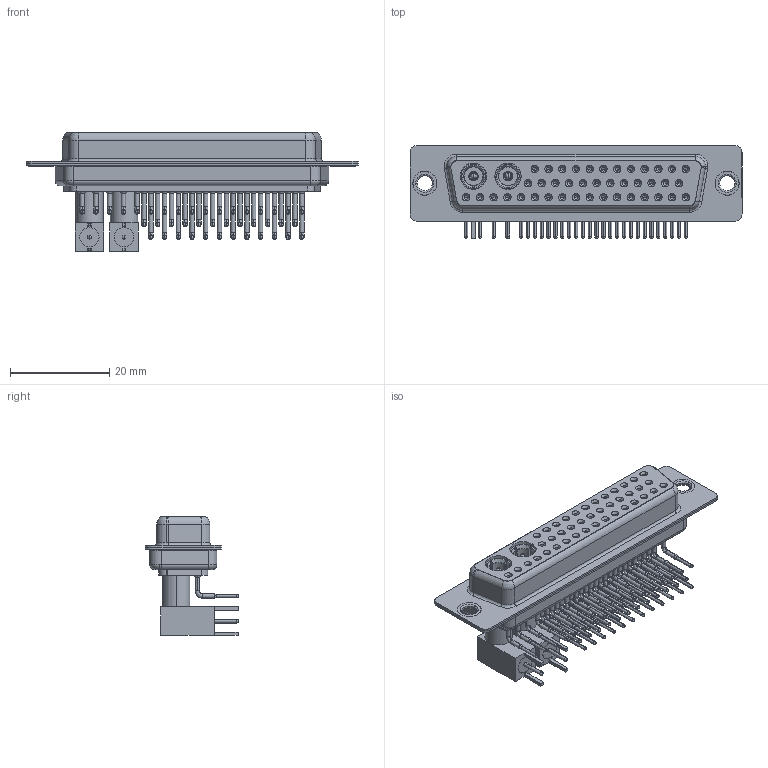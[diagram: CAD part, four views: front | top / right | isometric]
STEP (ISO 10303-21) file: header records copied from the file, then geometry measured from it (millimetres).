
FILE_DESCRIPTION (( 'STEP AP203' ), '1' );
FILE_NAME ('630-43W2240-7T1.STEP', '2022-06-09T19:07:29', ( '' ), ( '' ), 'SwSTEP 2.0', 'SolidWorks 2020', '' );
FILE_SCHEMA (( 'CONFIG_CONTROL_DESIGN' ));
Length unit declared in the file: millimetre
Products named in the file (16): 630Combo Housing_43W2; Locking Collar; Insulator RA Pin; 630Combo Thru Hole Rivet; Co-Ax Plug_RA 50; 630Combo Shell Rear_50 Contacts; 630-43W2240-7T1; 630Combo Shell Front_50 Contacts; RA Back Shell_50; Insulator Pin_Straight PC Tail; 630Combo Contact Row 3; 630Combo Contact Row 2_50 Contacts; Co-Ax Plug Assy_RA 50; Pin_RA 50; 630Combo Contact Row 1_50 Contacts
Assembly tree (60 placements, depth 3):
  630-43W2240-7T1
    630Combo Housing_43W2
    630Combo Shell Front_50 Contacts
    630Combo Shell Rear_50 Contacts
    630Combo Thru Hole Rivet  x2
    Co-Ax Plug Assy_RA 50
      Co-Ax Plug_RA 50
      Insulator Pin_Straight PC Tail
      Pin_RA 50
      Locking Collar
      RA Back Shell_50
      Insulator RA Pin
    Co-Ax Plug Assy_RA 50
      Co-Ax Plug_RA 50
      Insulator Pin_Straight PC Tail
      Pin_RA 50
      Locking Collar
      RA Back Shell_50
      Insulator RA Pin
    630Combo Contact Row 1_50 Contacts  x12
    630Combo Contact Row 2_50 Contacts  x12
    630Combo Contact Row 3  x17
Bounding box: 67 x 18.8 x 23.95 mm (x, y, z)
Volume: 7701.7 mm3; surface area: 17277.3 mm2
Topology: 58 solids, 58 shells, 2762 faces, 6940 edges, 4358 vertices
Faces by surface type: cylinder 1194, plane 816, cone 501, bspline 166, torus 77, sphere 8
Entity records: 34065 total; most frequent: DIRECTION 5913, CARTESIAN_POINT 5773, ORIENTED_EDGE 4842, AXIS2_PLACEMENT_3D 2476, EDGE_CURVE 2421, VERTEX_POINT 1543, CIRCLE 1365, EDGE_LOOP 1322
